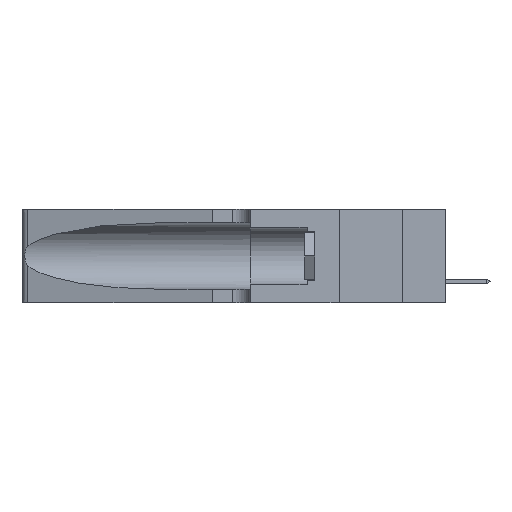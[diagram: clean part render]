
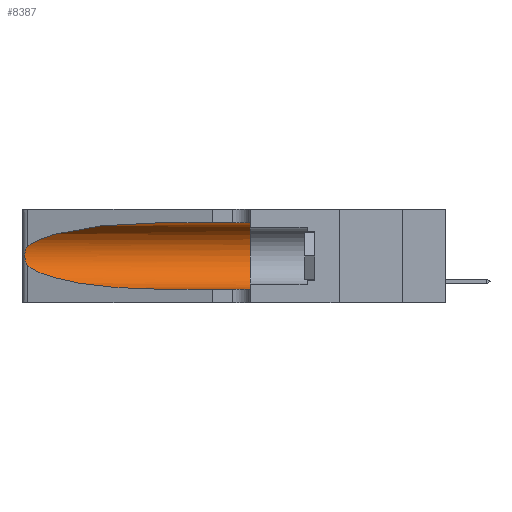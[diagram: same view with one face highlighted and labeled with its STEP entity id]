
A CAD part, left-side view. The second image highlights one B-rep face of the part: STEP entity #8387.
In plain terms, the highlighted cylindrical face has radius 3.308 mm (diameter 6.617 mm), a partial arc.
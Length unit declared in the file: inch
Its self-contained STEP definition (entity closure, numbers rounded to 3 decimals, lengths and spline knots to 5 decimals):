
#572 = CARTESIAN_POINT ( 'NONE',  ( 0.1305, 1.61858, 0.05475 ) ) ;
#1747 = CARTESIAN_POINT ( 'NONE',  ( 0.2373, 1.15595, 0.28018 ) ) ;
#2367 = ORIENTED_EDGE ( 'NONE', *, *, #14394, .T. ) ;
#2900 = CARTESIAN_POINT ( 'NONE',  ( 0.2373, 1.15595, 0.08982 ) ) ;
#4035 = CARTESIAN_POINT ( 'NONE',  ( 0.25487, 1.22718, 0.14631 ) ) ;
#4158 = CARTESIAN_POINT ( 'NONE',  ( 0.25787, 1.23484, 0.2124 ) ) ;
#4453 = EDGE_CURVE ( 'NONE', #6753, #33943, #19861, .T. ) ;
#6658 = CARTESIAN_POINT ( 'NONE',  ( 0.26018, 1.23835, 0.19895 ) ) ;
#6753 = VERTEX_POINT ( 'NONE', #10816 ) ;
#7045 = CARTESIAN_POINT ( 'NONE',  ( 0.25856, 1.23593, 0.16098 ) ) ;
#7618 = CARTESIAN_POINT ( 'NONE',  ( 0.1305, 0.72297, 0.31525 ) ) ;
#8387 = ADVANCED_FACE ( 'NONE', ( #31116 ), #12245, .F. ) ;
#8403 = CARTESIAN_POINT ( 'NONE',  ( 0.1305, 0.72297, 0.31525 ) ) ;
#8488 = DIRECTION ( 'NONE',  ( 0., 1., 0. ) ) ;
#8765 = CARTESIAN_POINT ( 'NONE',  ( 0.1305, 0.72297, 0.05475 ) ) ;
#10470 = LINE ( 'NONE', #27532, #14441 ) ;
#10512 = ORIENTED_EDGE ( 'NONE', *, *, #18625, .F. ) ;
#10816 = CARTESIAN_POINT ( 'NONE',  ( 0.1305, 0.35, 0.31525 ) ) ;
#11230 = AXIS2_PLACEMENT_3D ( 'NONE', #28232, #19328, #28360 ) ;
#11290 = VERTEX_POINT ( 'NONE', #8403 ) ;
#11561 = CARTESIAN_POINT ( 'NONE',  ( 0.25487, 1.22718, 0.14631 ) ) ;
#12245 = CYLINDRICAL_SURFACE ( 'NONE', #11230, 0.13025 ) ;
#12654 = CARTESIAN_POINT ( 'NONE',  ( 0.25639, 1.23184, 0.21858 ) ) ;
#13986 = EDGE_LOOP ( 'NONE', ( #24626, #2367, #25877, #30888, #35171, #10512 ) ) ;
#14394 = EDGE_CURVE ( 'NONE', #22763, #37040, #28868, .T. ) ;
#14441 = VECTOR ( 'NONE', #30322, 39.37008 ) ;
#15647 = CARTESIAN_POINT ( 'NONE',  ( 0.25639, 1.23186, 0.15144 ) ) ;
#18263 = CARTESIAN_POINT ( 'NONE',  ( 0.25555, 1.22993, 0.14849 ) ) ;
#18436 = CARTESIAN_POINT ( 'NONE',  ( 0.1305, 0.72297, 0.05475 ) ) ;
#18625 = EDGE_CURVE ( 'NONE', #11290, #6753, #10470, .T. ) ;
#19076 = CARTESIAN_POINT ( 'NONE',  ( 0.25487, 1.22718, 0.22369 ) ) ;
#19328 = DIRECTION ( 'NONE',  ( 0., -1., 0. ) ) ;
#19861 = CIRCLE ( 'NONE', #33979, 0.13025 ) ;
#20149 = VERTEX_POINT ( 'NONE', #18436 ) ;
#22669 = LINE ( 'NONE', #572, #36142 ) ;
#22763 = VERTEX_POINT ( 'NONE', #35343 ) ;
#24046 =( BOUNDED_CURVE ( )  B_SPLINE_CURVE ( 3, ( #7618, #33028, #1747, #19076 ),
 .UNSPECIFIED., .F., .F. ) 
 B_SPLINE_CURVE_WITH_KNOTS ( ( 4, 4 ),
 ( 1.5708, 2.84003 ),
 .UNSPECIFIED. ) 
 CURVE ( )  GEOMETRIC_REPRESENTATION_ITEM ( )  RATIONAL_B_SPLINE_CURVE ( ( 1., 0.87, 0.87, 1. ) ) 
 REPRESENTATION_ITEM ( '' )  );
#24060 = CARTESIAN_POINT ( 'NONE',  ( 0.26017, 1.23833, 0.17102 ) ) ;
#24187 = CARTESIAN_POINT ( 'NONE',  ( 0.26075, 1.23896, 0.19203 ) ) ;
#24626 = ORIENTED_EDGE ( 'NONE', *, *, #29737, .T. ) ;
#24899 = CARTESIAN_POINT ( 'NONE',  ( 0.1305, 0.35, 0.05475 ) ) ;
#25045 = EDGE_CURVE ( 'NONE', #37040, #20149, #33478, .T. ) ;
#25713 = EDGE_CURVE ( 'NONE', #20149, #33943, #22669, .T. ) ;
#25877 = ORIENTED_EDGE ( 'NONE', *, *, #25045, .T. ) ;
#27051 = CARTESIAN_POINT ( 'NONE',  ( 0.25487, 1.22718, 0.22369 ) ) ;
#27532 = CARTESIAN_POINT ( 'NONE',  ( 0.1305, 1.61858, 0.31525 ) ) ;
#28232 = CARTESIAN_POINT ( 'NONE',  ( 0.1305, 1.61858, 0.185 ) ) ;
#28360 = DIRECTION ( 'NONE',  ( 0., 0., -1. ) ) ;
#28868 = B_SPLINE_CURVE_WITH_KNOTS ( 'NONE', 3,
 ( #27051, #30088, #12654, #4158, #29829, #6658, #24187, #35337, #24060, #7045, #32710, #15647, #18263, #4035 ),
 .UNSPECIFIED., .F., .F.,
 ( 4, 2, 2, 2, 2, 2, 4 ),
 ( 0., 0.00027, 0.00053, 0.00107, 0.0016, 0.00187, 0.00214 ),
 .UNSPECIFIED. ) ;
#29737 = EDGE_CURVE ( 'NONE', #11290, #22763, #24046, .T. ) ;
#29829 = CARTESIAN_POINT ( 'NONE',  ( 0.25854, 1.2359, 0.20912 ) ) ;
#30088 = CARTESIAN_POINT ( 'NONE',  ( 0.25555, 1.22994, 0.2215 ) ) ;
#30322 = DIRECTION ( 'NONE',  ( 0., -1., 0. ) ) ;
#30888 = ORIENTED_EDGE ( 'NONE', *, *, #25713, .T. ) ;
#31116 = FACE_OUTER_BOUND ( 'NONE', #13986, .T. ) ;
#31573 = CARTESIAN_POINT ( 'NONE',  ( 0.18966, 0.96281, 0.05475 ) ) ;
#31691 = CARTESIAN_POINT ( 'NONE',  ( 0.25487, 1.22718, 0.14631 ) ) ;
#32004 = DIRECTION ( 'NONE',  ( 0., -1., 0. ) ) ;
#32710 = CARTESIAN_POINT ( 'NONE',  ( 0.25789, 1.23486, 0.15765 ) ) ;
#33028 = CARTESIAN_POINT ( 'NONE',  ( 0.18966, 0.96281, 0.31525 ) ) ;
#33478 =( BOUNDED_CURVE ( )  B_SPLINE_CURVE ( 3, ( #31691, #2900, #31573, #8765 ),
 .UNSPECIFIED., .F., .F. ) 
 B_SPLINE_CURVE_WITH_KNOTS ( ( 4, 4 ),
 ( 3.44316, 4.71239 ),
 .UNSPECIFIED. ) 
 CURVE ( )  GEOMETRIC_REPRESENTATION_ITEM ( )  RATIONAL_B_SPLINE_CURVE ( ( 1., 0.87, 0.87, 1. ) ) 
 REPRESENTATION_ITEM ( '' )  );
#33943 = VERTEX_POINT ( 'NONE', #24899 ) ;
#33979 = AXIS2_PLACEMENT_3D ( 'NONE', #34529, #8488, #34656 ) ;
#34529 = CARTESIAN_POINT ( 'NONE',  ( 0.1305, 0.35, 0.185 ) ) ;
#34656 = DIRECTION ( 'NONE',  ( 0., 0., 1. ) ) ;
#35171 = ORIENTED_EDGE ( 'NONE', *, *, #4453, .F. ) ;
#35337 = CARTESIAN_POINT ( 'NONE',  ( 0.26075, 1.23896, 0.178 ) ) ;
#35343 = CARTESIAN_POINT ( 'NONE',  ( 0.25487, 1.22718, 0.22369 ) ) ;
#36142 = VECTOR ( 'NONE', #32004, 39.37008 ) ;
#37040 = VERTEX_POINT ( 'NONE', #11561 ) ;
